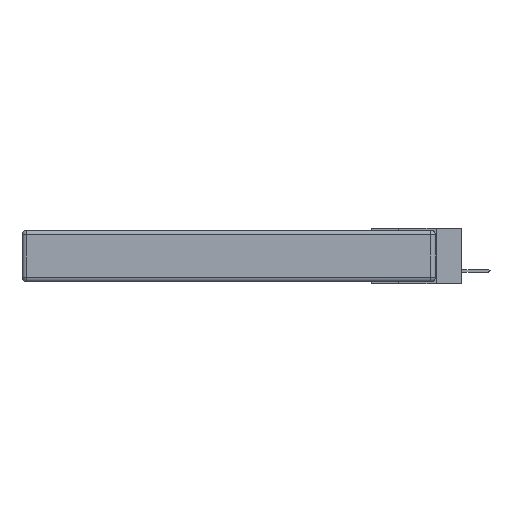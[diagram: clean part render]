
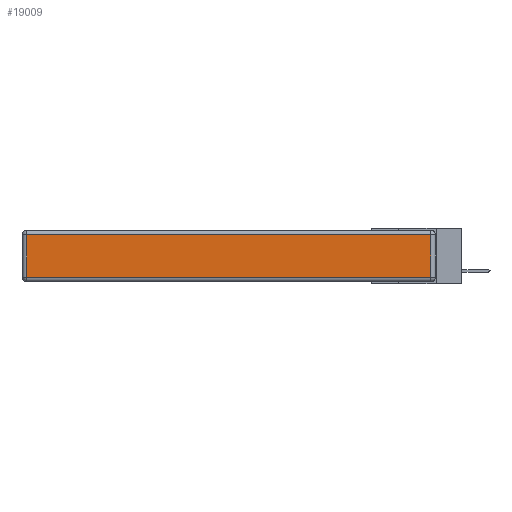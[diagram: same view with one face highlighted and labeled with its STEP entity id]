
A CAD part, left-side view. The second image highlights one B-rep face of the part: STEP entity #19009.
In plain terms, the highlighted planar face has unit normal (-1, 0, 0).
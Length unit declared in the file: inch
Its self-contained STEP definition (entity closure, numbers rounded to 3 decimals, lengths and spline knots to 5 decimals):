
#708 = VERTEX_POINT ( 'NONE', #3456 ) ;
#1185 = DIRECTION ( 'NONE',  ( -1., 0., 0. ) ) ;
#2638 = EDGE_CURVE ( 'NONE', #708, #12025, #18400, .T. ) ;
#3050 = DIRECTION ( 'NONE',  ( 0., 1., 0. ) ) ;
#3456 = CARTESIAN_POINT ( 'NONE',  ( 0., 2.72, -0.03 ) ) ;
#3651 = VECTOR ( 'NONE', #18431, 39.37008 ) ;
#5492 = CARTESIAN_POINT ( 'NONE',  ( 0., 0., -0.313 ) ) ;
#5578 = DIRECTION ( 'NONE',  ( 0., 0., -1. ) ) ;
#5597 = EDGE_LOOP ( 'NONE', ( #19965, #15662, #26632, #22939 ) ) ;
#5985 = VERTEX_POINT ( 'NONE', #26055 ) ;
#6438 = FACE_OUTER_BOUND ( 'NONE', #5597, .T. ) ;
#7639 = EDGE_CURVE ( 'NONE', #12025, #26684, #26198, .T. ) ;
#8375 = CARTESIAN_POINT ( 'NONE',  ( 0., 0.03, -0.343 ) ) ;
#9696 = CARTESIAN_POINT ( 'NONE',  ( 0., 2.72, -0.343 ) ) ;
#10221 = LINE ( 'NONE', #11504, #26503 ) ;
#11504 = CARTESIAN_POINT ( 'NONE',  ( 0., 2.75, -0.03 ) ) ;
#12025 = VERTEX_POINT ( 'NONE', #27244 ) ;
#12553 = DIRECTION ( 'NONE',  ( 0., 0., 1. ) ) ;
#14297 = CARTESIAN_POINT ( 'NONE',  ( 0., 0.03, -0.313 ) ) ;
#15662 = ORIENTED_EDGE ( 'NONE', *, *, #18885, .T. ) ;
#18400 = LINE ( 'NONE', #9696, #25638 ) ;
#18431 = DIRECTION ( 'NONE',  ( 0., -1., 0. ) ) ;
#18885 = EDGE_CURVE ( 'NONE', #26684, #5985, #25031, .T. ) ;
#19009 = ADVANCED_FACE ( 'NONE', ( #6438 ), #25840, .T. ) ;
#19341 = CARTESIAN_POINT ( 'NONE',  ( 0., 0., -0.343 ) ) ;
#19965 = ORIENTED_EDGE ( 'NONE', *, *, #7639, .T. ) ;
#20732 = VECTOR ( 'NONE', #21411, 39.37008 ) ;
#21411 = DIRECTION ( 'NONE',  ( 0., 0., 1. ) ) ;
#22939 = ORIENTED_EDGE ( 'NONE', *, *, #2638, .T. ) ;
#23725 = AXIS2_PLACEMENT_3D ( 'NONE', #19341, #1185, #12553 ) ;
#25031 = LINE ( 'NONE', #8375, #20732 ) ;
#25638 = VECTOR ( 'NONE', #5578, 39.37008 ) ;
#25840 = PLANE ( 'NONE',  #23725 ) ;
#26055 = CARTESIAN_POINT ( 'NONE',  ( 0., 0.03, -0.03 ) ) ;
#26198 = LINE ( 'NONE', #5492, #3651 ) ;
#26503 = VECTOR ( 'NONE', #3050, 39.37008 ) ;
#26632 = ORIENTED_EDGE ( 'NONE', *, *, #27072, .T. ) ;
#26684 = VERTEX_POINT ( 'NONE', #14297 ) ;
#27072 = EDGE_CURVE ( 'NONE', #5985, #708, #10221, .T. ) ;
#27244 = CARTESIAN_POINT ( 'NONE',  ( 0., 2.72, -0.313 ) ) ;
